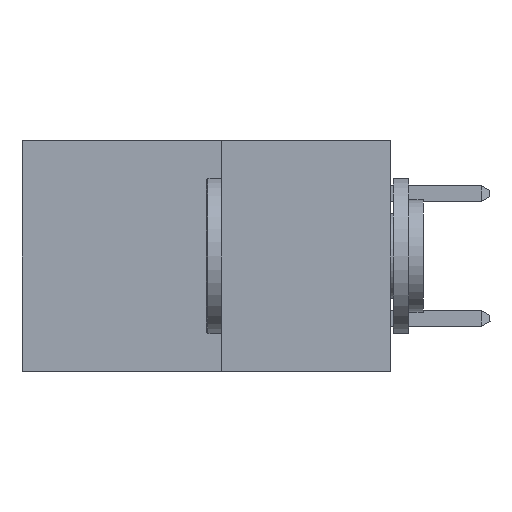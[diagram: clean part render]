
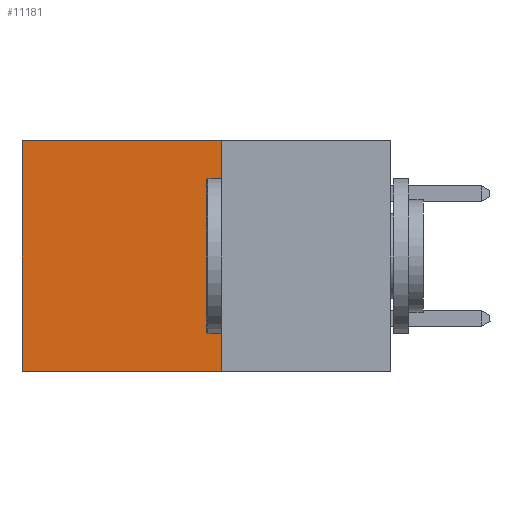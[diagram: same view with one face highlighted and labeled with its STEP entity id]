
A CAD part, left-side view. The second image highlights one B-rep face of the part: STEP entity #11181.
In plain terms, the highlighted planar face has unit normal (-1, 0, 0).
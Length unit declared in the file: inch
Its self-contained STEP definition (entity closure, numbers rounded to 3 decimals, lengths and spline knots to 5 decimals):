
#2808 = VERTEX_POINT ( 'NONE', #14677 ) ;
#3656 = DIRECTION ( 'NONE',  ( 0., 1., 0. ) ) ;
#3801 = DIRECTION ( 'NONE',  ( 0., 1., 0. ) ) ;
#5739 = DIRECTION ( 'NONE',  ( 1., 0., 0. ) ) ;
#5940 = EDGE_LOOP ( 'NONE', ( #8379, #24217, #10251, #22498 ) ) ;
#8311 = CARTESIAN_POINT ( 'NONE',  ( 0.277, 0.27, -0.37 ) ) ;
#8379 = ORIENTED_EDGE ( 'NONE', *, *, #30348, .T. ) ;
#8804 = CARTESIAN_POINT ( 'NONE',  ( 0.277, 0.27, 0. ) ) ;
#9168 = LINE ( 'NONE', #30079, #23226 ) ;
#9900 = DIRECTION ( 'NONE',  ( 0., 0., -1. ) ) ;
#10251 = ORIENTED_EDGE ( 'NONE', *, *, #13449, .F. ) ;
#11181 = ADVANCED_FACE ( 'NONE', ( #13421 ), #21555, .F. ) ;
#11364 = EDGE_CURVE ( 'NONE', #16699, #26623, #15942, .T. ) ;
#11591 = DIRECTION ( 'NONE',  ( 0., 0., -1. ) ) ;
#12071 = CARTESIAN_POINT ( 'NONE',  ( 0.277, 0.27, -0.37 ) ) ;
#12975 = CARTESIAN_POINT ( 'NONE',  ( 0.277, 0.59, -0.37 ) ) ;
#13421 = FACE_OUTER_BOUND ( 'NONE', #5940, .T. ) ;
#13449 = EDGE_CURVE ( 'NONE', #14628, #16699, #33955, .T. ) ;
#14628 = VERTEX_POINT ( 'NONE', #8804 ) ;
#14677 = CARTESIAN_POINT ( 'NONE',  ( 0.277, 0.59, 0. ) ) ;
#15942 = LINE ( 'NONE', #27456, #16757 ) ;
#16699 = VERTEX_POINT ( 'NONE', #12071 ) ;
#16757 = VECTOR ( 'NONE', #3656, 39.37008 ) ;
#16894 = VECTOR ( 'NONE', #3801, 39.37008 ) ;
#20739 = VECTOR ( 'NONE', #9900, 39.37008 ) ;
#21555 = PLANE ( 'NONE',  #25844 ) ;
#22498 = ORIENTED_EDGE ( 'NONE', *, *, #27007, .T. ) ;
#23226 = VECTOR ( 'NONE', #11591, 39.37008 ) ;
#24217 = ORIENTED_EDGE ( 'NONE', *, *, #11364, .F. ) ;
#24246 = DIRECTION ( 'NONE',  ( 0., 0., -1. ) ) ;
#24787 = LINE ( 'NONE', #24970, #16894 ) ;
#24970 = CARTESIAN_POINT ( 'NONE',  ( 0.277, 0.27, 0. ) ) ;
#25844 = AXIS2_PLACEMENT_3D ( 'NONE', #8311, #5739, #24246 ) ;
#26623 = VERTEX_POINT ( 'NONE', #12975 ) ;
#27007 = EDGE_CURVE ( 'NONE', #14628, #2808, #24787, .T. ) ;
#27456 = CARTESIAN_POINT ( 'NONE',  ( 0.277, 0.27, -0.37 ) ) ;
#30079 = CARTESIAN_POINT ( 'NONE',  ( 0.277, 0.59, -0.37 ) ) ;
#30348 = EDGE_CURVE ( 'NONE', #2808, #26623, #9168, .T. ) ;
#33569 = CARTESIAN_POINT ( 'NONE',  ( 0.277, 0.27, -0.37 ) ) ;
#33955 = LINE ( 'NONE', #33569, #20739 ) ;
